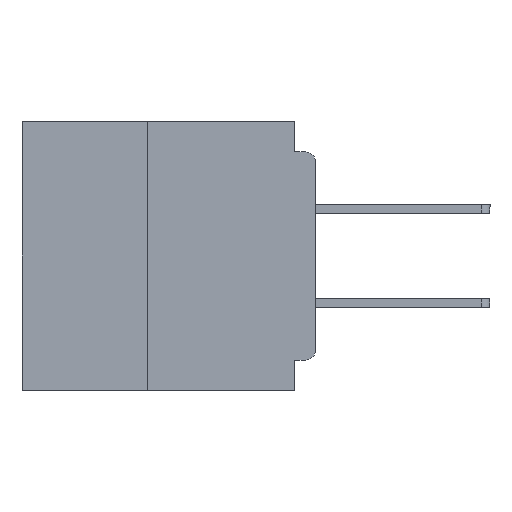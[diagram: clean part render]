
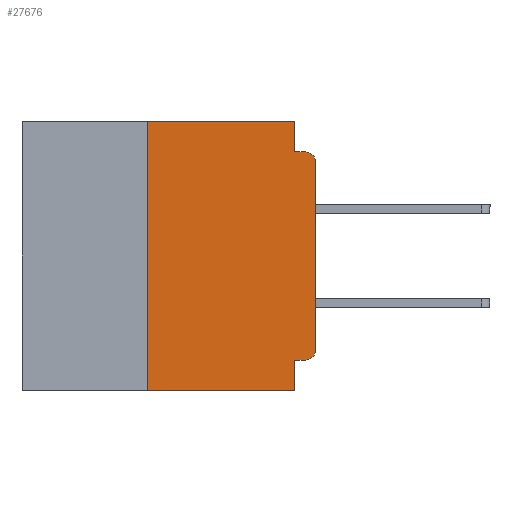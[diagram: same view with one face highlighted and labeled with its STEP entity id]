
A CAD part, left-side view. The second image highlights one B-rep face of the part: STEP entity #27676.
In plain terms, the highlighted planar face has unit normal (-1, 0, 0).
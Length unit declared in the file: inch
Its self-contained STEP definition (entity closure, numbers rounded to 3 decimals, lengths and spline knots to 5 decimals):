
#168 = CARTESIAN_POINT ( 'NONE',  ( 0., 0.25, 0. ) ) ;
#2145 = VERTEX_POINT ( 'NONE', #16468 ) ;
#2186 = VECTOR ( 'NONE', #22743, 39.37008 ) ;
#3029 = CIRCLE ( 'NONE', #8983, 0.015 ) ;
#3428 = EDGE_CURVE ( 'NONE', #9829, #25193, #27404, .T. ) ;
#4397 = VECTOR ( 'NONE', #26319, 39.37008 ) ;
#4650 = VERTEX_POINT ( 'NONE', #6378 ) ;
#4763 = AXIS2_PLACEMENT_3D ( 'NONE', #21843, #21676, #21544 ) ;
#5440 = DIRECTION ( 'NONE',  ( 0., 1., 0. ) ) ;
#5767 = CARTESIAN_POINT ( 'NONE',  ( 0., 0., 0. ) ) ;
#5864 = VECTOR ( 'NONE', #40999, 39.37008 ) ;
#6378 = CARTESIAN_POINT ( 'NONE',  ( 0., 0.031, 0. ) ) ;
#6388 = LINE ( 'NONE', #14291, #41725 ) ;
#6442 = DIRECTION ( 'NONE',  ( -1., 0., 0. ) ) ;
#6903 = VECTOR ( 'NONE', #8793, 39.37008 ) ;
#7025 = ORIENTED_EDGE ( 'NONE', *, *, #32682, .F. ) ;
#7520 = EDGE_CURVE ( 'NONE', #19393, #31552, #3029, .T. ) ;
#8793 = DIRECTION ( 'NONE',  ( 0., -1., 0. ) ) ;
#8915 = LINE ( 'NONE', #21471, #44105 ) ;
#8983 = AXIS2_PLACEMENT_3D ( 'NONE', #26966, #6442, #30439 ) ;
#9104 = ORIENTED_EDGE ( 'NONE', *, *, #25780, .T. ) ;
#9292 = ORIENTED_EDGE ( 'NONE', *, *, #16669, .F. ) ;
#9829 = VERTEX_POINT ( 'NONE', #29235 ) ;
#10807 = ORIENTED_EDGE ( 'NONE', *, *, #3428, .T. ) ;
#11474 = LINE ( 'NONE', #32914, #2186 ) ;
#12587 = LINE ( 'NONE', #5767, #4397 ) ;
#14291 = CARTESIAN_POINT ( 'NONE',  ( 0., 0.031, -0.4 ) ) ;
#14397 = CARTESIAN_POINT ( 'NONE',  ( 0., 0.437, 0. ) ) ;
#14572 = CARTESIAN_POINT ( 'NONE',  ( 0., 0., -0.34 ) ) ;
#15132 = ORIENTED_EDGE ( 'NONE', *, *, #39540, .F. ) ;
#15299 = ORIENTED_EDGE ( 'NONE', *, *, #27932, .F. ) ;
#15614 = CARTESIAN_POINT ( 'NONE',  ( 0., 0., -0.355 ) ) ;
#16154 = LINE ( 'NONE', #18991, #6903 ) ;
#16468 = CARTESIAN_POINT ( 'NONE',  ( 0., 0.031, -0.355 ) ) ;
#16669 = EDGE_CURVE ( 'NONE', #2145, #32372, #6388, .T. ) ;
#16915 = CARTESIAN_POINT ( 'NONE',  ( 0., 0.015, -0.355 ) ) ;
#17326 = VECTOR ( 'NONE', #5440, 39.37008 ) ;
#17519 = EDGE_CURVE ( 'NONE', #33332, #4650, #16154, .T. ) ;
#17991 = EDGE_LOOP ( 'NONE', ( #29270, #10807, #39114, #15132, #43352, #7025, #9104, #9292, #15299, #29223 ) ) ;
#18991 = CARTESIAN_POINT ( 'NONE',  ( 0., 0.437, 0. ) ) ;
#19393 = VERTEX_POINT ( 'NONE', #16915 ) ;
#19922 = VERTEX_POINT ( 'NONE', #30144 ) ;
#21237 = DIRECTION ( 'NONE',  ( 0., 0., -1. ) ) ;
#21471 = CARTESIAN_POINT ( 'NONE',  ( 0., 0., -0.045 ) ) ;
#21544 = DIRECTION ( 'NONE',  ( 0., 0., -1. ) ) ;
#21676 = DIRECTION ( 'NONE',  ( -1., 0., 0. ) ) ;
#21843 = CARTESIAN_POINT ( 'NONE',  ( 0., 0.015, -0.06 ) ) ;
#21931 = EDGE_CURVE ( 'NONE', #31552, #9829, #12587, .T. ) ;
#22348 = VERTEX_POINT ( 'NONE', #38544 ) ;
#22743 = DIRECTION ( 'NONE',  ( 0., 0., -1. ) ) ;
#25193 = VERTEX_POINT ( 'NONE', #27890 ) ;
#25299 = EDGE_CURVE ( 'NONE', #19922, #25193, #8915, .T. ) ;
#25780 = EDGE_CURVE ( 'NONE', #22348, #32372, #35059, .T. ) ;
#25973 = VECTOR ( 'NONE', #30712, 39.37008 ) ;
#26319 = DIRECTION ( 'NONE',  ( 0., 0., 1. ) ) ;
#26966 = CARTESIAN_POINT ( 'NONE',  ( 0., 0.015, -0.34 ) ) ;
#27404 = CIRCLE ( 'NONE', #4763, 0.015 ) ;
#27676 = ADVANCED_FACE ( 'NONE', ( #36027 ), #38271, .F. ) ;
#27890 = CARTESIAN_POINT ( 'NONE',  ( 0., 0.015, -0.045 ) ) ;
#27932 = EDGE_CURVE ( 'NONE', #19393, #2145, #35465, .T. ) ;
#29223 = ORIENTED_EDGE ( 'NONE', *, *, #7520, .T. ) ;
#29235 = CARTESIAN_POINT ( 'NONE',  ( 0., 0., -0.06 ) ) ;
#29270 = ORIENTED_EDGE ( 'NONE', *, *, #21931, .T. ) ;
#30144 = CARTESIAN_POINT ( 'NONE',  ( 0., 0.031, -0.045 ) ) ;
#30439 = DIRECTION ( 'NONE',  ( 0., 0., -1. ) ) ;
#30712 = DIRECTION ( 'NONE',  ( 0., -1., 0. ) ) ;
#31552 = VERTEX_POINT ( 'NONE', #14572 ) ;
#32372 = VERTEX_POINT ( 'NONE', #39406 ) ;
#32682 = EDGE_CURVE ( 'NONE', #22348, #33332, #33222, .T. ) ;
#32914 = CARTESIAN_POINT ( 'NONE',  ( 0., 0.031, 0. ) ) ;
#33222 = LINE ( 'NONE', #37572, #5864 ) ;
#33332 = VERTEX_POINT ( 'NONE', #168 ) ;
#35059 = LINE ( 'NONE', #40547, #25973 ) ;
#35465 = LINE ( 'NONE', #15614, #17326 ) ;
#36027 = FACE_OUTER_BOUND ( 'NONE', #17991, .T. ) ;
#37535 = AXIS2_PLACEMENT_3D ( 'NONE', #14397, #41669, #21237 ) ;
#37572 = CARTESIAN_POINT ( 'NONE',  ( 0., 0.25, -0.4 ) ) ;
#38141 = DIRECTION ( 'NONE',  ( 0., 0., -1. ) ) ;
#38271 = PLANE ( 'NONE',  #37535 ) ;
#38544 = CARTESIAN_POINT ( 'NONE',  ( 0., 0.25, -0.4 ) ) ;
#39114 = ORIENTED_EDGE ( 'NONE', *, *, #25299, .F. ) ;
#39406 = CARTESIAN_POINT ( 'NONE',  ( 0., 0.031, -0.4 ) ) ;
#39540 = EDGE_CURVE ( 'NONE', #4650, #19922, #11474, .T. ) ;
#40547 = CARTESIAN_POINT ( 'NONE',  ( 0., 0.437, -0.4 ) ) ;
#40999 = DIRECTION ( 'NONE',  ( 0., 0., 1. ) ) ;
#41669 = DIRECTION ( 'NONE',  ( 1., 0., 0. ) ) ;
#41725 = VECTOR ( 'NONE', #38141, 39.37008 ) ;
#42068 = DIRECTION ( 'NONE',  ( 0., -1., 0. ) ) ;
#43352 = ORIENTED_EDGE ( 'NONE', *, *, #17519, .F. ) ;
#44105 = VECTOR ( 'NONE', #42068, 39.37008 ) ;
